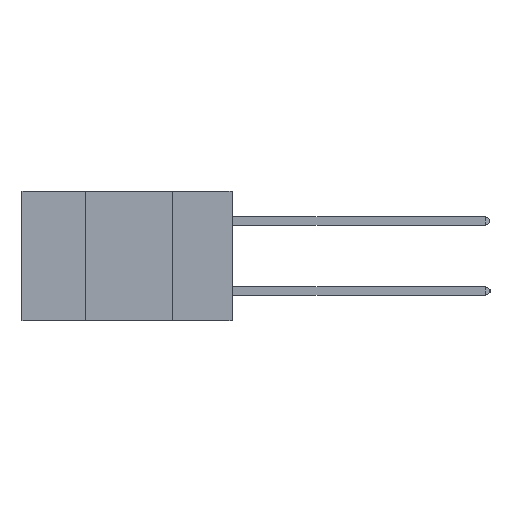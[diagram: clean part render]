
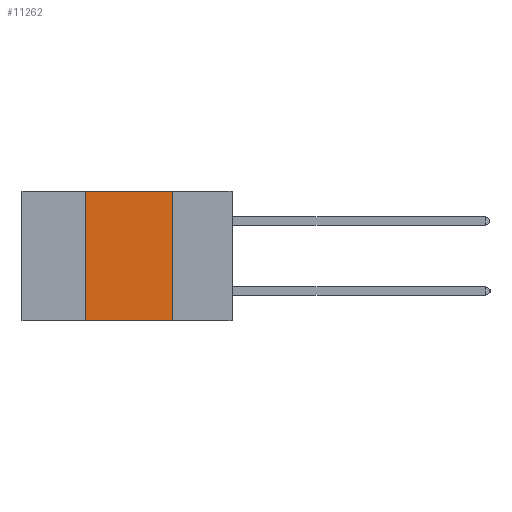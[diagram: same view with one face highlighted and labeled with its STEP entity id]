
A CAD part, left-side view. The second image highlights one B-rep face of the part: STEP entity #11262.
In plain terms, the highlighted planar face has unit normal (-1, 0, 0).
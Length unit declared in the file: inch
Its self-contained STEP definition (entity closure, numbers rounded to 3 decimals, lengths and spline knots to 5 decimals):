
#236 = VECTOR ( 'NONE', #4752, 39.37008 ) ;
#273 = CARTESIAN_POINT ( 'NONE',  ( 0., 0.6, -0.37 ) ) ;
#772 = DIRECTION ( 'NONE',  ( 0., -1., 0. ) ) ;
#1288 = VERTEX_POINT ( 'NONE', #1534 ) ;
#1534 = CARTESIAN_POINT ( 'NONE',  ( 0., 0.17, -0.37 ) ) ;
#2071 = EDGE_CURVE ( 'NONE', #5997, #4509, #13400, .T. ) ;
#2205 = CARTESIAN_POINT ( 'NONE',  ( 0., 0.42, -0.37 ) ) ;
#2620 = DIRECTION ( 'NONE',  ( 0., 0., -1. ) ) ;
#3284 = LINE ( 'NONE', #273, #236 ) ;
#3878 = VECTOR ( 'NONE', #9030, 39.37008 ) ;
#4509 = VERTEX_POINT ( 'NONE', #13534 ) ;
#4752 = DIRECTION ( 'NONE',  ( 0., -1., 0. ) ) ;
#5043 = VERTEX_POINT ( 'NONE', #8385 ) ;
#5898 = CARTESIAN_POINT ( 'NONE',  ( 0., 0.17, 0. ) ) ;
#5997 = VERTEX_POINT ( 'NONE', #2205 ) ;
#6157 = AXIS2_PLACEMENT_3D ( 'NONE', #8316, #9465, #2620 ) ;
#7155 = PLANE ( 'NONE',  #6157 ) ;
#8316 = CARTESIAN_POINT ( 'NONE',  ( 0., 0.6, 0. ) ) ;
#8385 = CARTESIAN_POINT ( 'NONE',  ( 0., 0.17, 0. ) ) ;
#8837 = EDGE_CURVE ( 'NONE', #5997, #1288, #3284, .T. ) ;
#8976 = ORIENTED_EDGE ( 'NONE', *, *, #11192, .F. ) ;
#9030 = DIRECTION ( 'NONE',  ( 0., 0., 1. ) ) ;
#9088 = LINE ( 'NONE', #5898, #12678 ) ;
#9465 = DIRECTION ( 'NONE',  ( 1., 0., 0. ) ) ;
#9634 = FACE_OUTER_BOUND ( 'NONE', #10044, .T. ) ;
#9861 = LINE ( 'NONE', #14496, #12197 ) ;
#10010 = EDGE_CURVE ( 'NONE', #4509, #5043, #9861, .T. ) ;
#10044 = EDGE_LOOP ( 'NONE', ( #8976, #14016, #12180, #10791 ) ) ;
#10791 = ORIENTED_EDGE ( 'NONE', *, *, #8837, .T. ) ;
#11192 = EDGE_CURVE ( 'NONE', #5043, #1288, #9088, .T. ) ;
#11262 = ADVANCED_FACE ( 'NONE', ( #9634 ), #7155, .F. ) ;
#12180 = ORIENTED_EDGE ( 'NONE', *, *, #2071, .F. ) ;
#12197 = VECTOR ( 'NONE', #772, 39.37008 ) ;
#12410 = CARTESIAN_POINT ( 'NONE',  ( 0., 0.42, 0. ) ) ;
#12644 = DIRECTION ( 'NONE',  ( 0., 0., -1. ) ) ;
#12678 = VECTOR ( 'NONE', #12644, 39.37008 ) ;
#13400 = LINE ( 'NONE', #12410, #3878 ) ;
#13534 = CARTESIAN_POINT ( 'NONE',  ( 0., 0.42, 0. ) ) ;
#14016 = ORIENTED_EDGE ( 'NONE', *, *, #10010, .F. ) ;
#14496 = CARTESIAN_POINT ( 'NONE',  ( 0., 0.6, 0. ) ) ;
